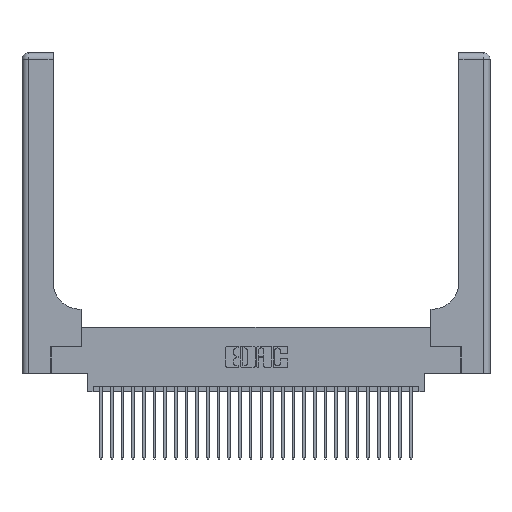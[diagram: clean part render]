
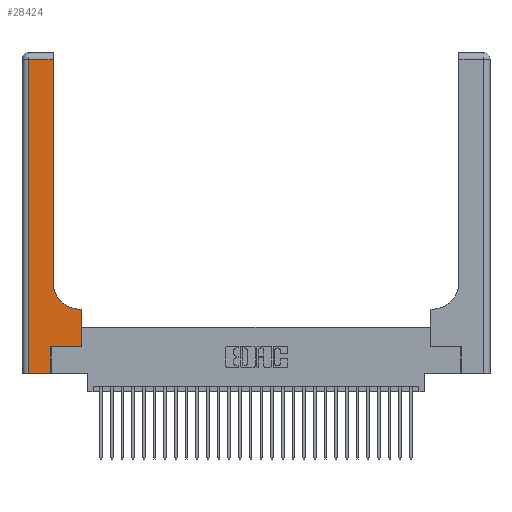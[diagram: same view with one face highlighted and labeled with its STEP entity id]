
A CAD part, top view. The second image highlights one B-rep face of the part: STEP entity #28424.
In plain terms, the highlighted planar face has unit normal (0, 0, 1).
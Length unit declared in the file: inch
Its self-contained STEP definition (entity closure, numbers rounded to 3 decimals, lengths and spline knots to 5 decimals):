
#92 = VERTEX_POINT ( 'NONE', #13784 ) ;
#136 = CARTESIAN_POINT ( 'NONE',  ( 0.269, 0.25, 0.37 ) ) ;
#447 = VERTEX_POINT ( 'NONE', #30286 ) ;
#609 = EDGE_CURVE ( 'NONE', #15232, #30178, #12545, .T. ) ;
#1901 = DIRECTION ( 'NONE',  ( 0., 1., 0. ) ) ;
#2073 = ORIENTED_EDGE ( 'NONE', *, *, #29675, .T. ) ;
#2083 = DIRECTION ( 'NONE',  ( 0., 0., -1. ) ) ;
#2339 = VECTOR ( 'NONE', #14311, 39.37008 ) ;
#2835 = CARTESIAN_POINT ( 'NONE',  ( 0.2915, 2.94, 0.37 ) ) ;
#2836 = CARTESIAN_POINT ( 'NONE',  ( 0.5415, 0.6, 0.37 ) ) ;
#3377 = VERTEX_POINT ( 'NONE', #2835 ) ;
#3553 = VECTOR ( 'NONE', #27394, 39.37008 ) ;
#3770 = EDGE_CURVE ( 'NONE', #3377, #25226, #26391, .T. ) ;
#6080 = DIRECTION ( 'NONE',  ( 0., 1., 0. ) ) ;
#6403 = ORIENTED_EDGE ( 'NONE', *, *, #609, .T. ) ;
#6567 = EDGE_CURVE ( 'NONE', #25226, #447, #17151, .T. ) ;
#7289 = DIRECTION ( 'NONE',  ( -1., 0., 0. ) ) ;
#7904 = EDGE_CURVE ( 'NONE', #30178, #3377, #18935, .T. ) ;
#8367 = ORIENTED_EDGE ( 'NONE', *, *, #29304, .T. ) ;
#8512 = CARTESIAN_POINT ( 'NONE',  ( 0.2915, 0.85, 0.37 ) ) ;
#8802 = CARTESIAN_POINT ( 'NONE',  ( 0.06, 3., 0.37 ) ) ;
#9872 = LINE ( 'NONE', #23309, #30198 ) ;
#9900 = DIRECTION ( 'NONE',  ( -1., 0., 0. ) ) ;
#10522 = EDGE_LOOP ( 'NONE', ( #23182, #24693, #17347, #2073, #11181, #13396, #16166, #8367, #6403 ) ) ;
#10738 = LINE ( 'NONE', #136, #22571 ) ;
#11181 = ORIENTED_EDGE ( 'NONE', *, *, #12569, .T. ) ;
#12033 = DIRECTION ( 'NONE',  ( 1., 0., 0. ) ) ;
#12545 = CIRCLE ( 'NONE', #21273, 0.25 ) ;
#12569 = EDGE_CURVE ( 'NONE', #92, #13526, #21305, .T. ) ;
#12653 = VECTOR ( 'NONE', #1901, 39.37008 ) ;
#13396 = ORIENTED_EDGE ( 'NONE', *, *, #18031, .T. ) ;
#13486 = CARTESIAN_POINT ( 'NONE',  ( 0.269, 0.25, 0.37 ) ) ;
#13526 = VERTEX_POINT ( 'NONE', #13486 ) ;
#13591 = EDGE_CURVE ( 'NONE', #19599, #28358, #9872, .T. ) ;
#13765 = DIRECTION ( 'NONE',  ( 1., 0., 0. ) ) ;
#13784 = CARTESIAN_POINT ( 'NONE',  ( 0.269, 0., 0.37 ) ) ;
#13886 = DIRECTION ( 'NONE',  ( 0., 1., 0. ) ) ;
#14311 = DIRECTION ( 'NONE',  ( 1., 0., 0. ) ) ;
#14967 = CARTESIAN_POINT ( 'NONE',  ( 0.269, 0., 0.37 ) ) ;
#15232 = VERTEX_POINT ( 'NONE', #2836 ) ;
#15961 = DIRECTION ( 'NONE',  ( -1., 0., 0. ) ) ;
#15968 = CARTESIAN_POINT ( 'NONE',  ( 0.2915, 3., 0.37 ) ) ;
#16145 = CARTESIAN_POINT ( 'NONE',  ( 0.5415, 0.85, 0.37 ) ) ;
#16166 = ORIENTED_EDGE ( 'NONE', *, *, #13591, .T. ) ;
#16838 = AXIS2_PLACEMENT_3D ( 'NONE', #18334, #25674, #15961 ) ;
#17151 = LINE ( 'NONE', #8802, #3553 ) ;
#17347 = ORIENTED_EDGE ( 'NONE', *, *, #6567, .T. ) ;
#18031 = EDGE_CURVE ( 'NONE', #13526, #19599, #10738, .T. ) ;
#18334 = CARTESIAN_POINT ( 'NONE',  ( 0., 3., 0.37 ) ) ;
#18935 = LINE ( 'NONE', #15968, #12653 ) ;
#19599 = VERTEX_POINT ( 'NONE', #28768 ) ;
#21273 = AXIS2_PLACEMENT_3D ( 'NONE', #16145, #2083, #13765 ) ;
#21305 = LINE ( 'NONE', #14967, #23862 ) ;
#22571 = VECTOR ( 'NONE', #12033, 39.37008 ) ;
#23121 = CARTESIAN_POINT ( 'NONE',  ( 0., 2.94, 0.37 ) ) ;
#23182 = ORIENTED_EDGE ( 'NONE', *, *, #7904, .T. ) ;
#23208 = PLANE ( 'NONE',  #16838 ) ;
#23309 = CARTESIAN_POINT ( 'NONE',  ( 0.5585, 0.25, 0.37 ) ) ;
#23862 = VECTOR ( 'NONE', #6080, 39.37008 ) ;
#24170 = VECTOR ( 'NONE', #7289, 39.37008 ) ;
#24693 = ORIENTED_EDGE ( 'NONE', *, *, #3770, .T. ) ;
#25226 = VERTEX_POINT ( 'NONE', #29643 ) ;
#25272 = CARTESIAN_POINT ( 'NONE',  ( 0.5585, 0.6, 0.37 ) ) ;
#25674 = DIRECTION ( 'NONE',  ( 0., 0., -1. ) ) ;
#25993 = CARTESIAN_POINT ( 'NONE',  ( 0., 0., 0.37 ) ) ;
#26391 = LINE ( 'NONE', #23121, #24170 ) ;
#26521 = CARTESIAN_POINT ( 'NONE',  ( 0.2915, 0.6, 0.37 ) ) ;
#27394 = DIRECTION ( 'NONE',  ( 0., -1., 0. ) ) ;
#28171 = VECTOR ( 'NONE', #9900, 39.37008 ) ;
#28358 = VERTEX_POINT ( 'NONE', #25272 ) ;
#28424 = ADVANCED_FACE ( 'NONE', ( #29347 ), #23208, .F. ) ;
#28768 = CARTESIAN_POINT ( 'NONE',  ( 0.5585, 0.25, 0.37 ) ) ;
#29259 = LINE ( 'NONE', #26521, #28171 ) ;
#29304 = EDGE_CURVE ( 'NONE', #28358, #15232, #29259, .T. ) ;
#29347 = FACE_OUTER_BOUND ( 'NONE', #10522, .T. ) ;
#29643 = CARTESIAN_POINT ( 'NONE',  ( 0.06, 2.94, 0.37 ) ) ;
#29675 = EDGE_CURVE ( 'NONE', #447, #92, #30360, .T. ) ;
#30178 = VERTEX_POINT ( 'NONE', #8512 ) ;
#30198 = VECTOR ( 'NONE', #13886, 39.37008 ) ;
#30286 = CARTESIAN_POINT ( 'NONE',  ( 0.06, 0., 0.37 ) ) ;
#30360 = LINE ( 'NONE', #25993, #2339 ) ;
